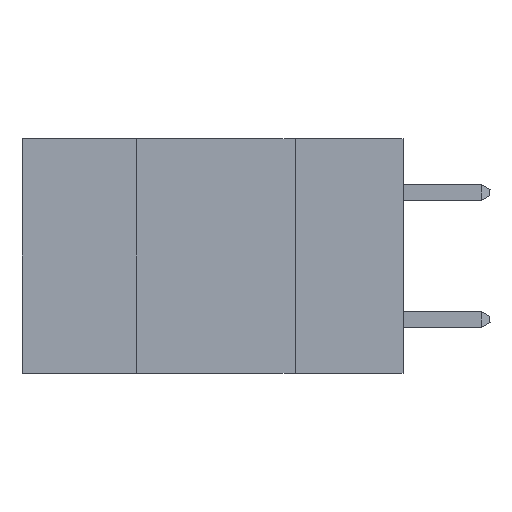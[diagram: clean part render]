
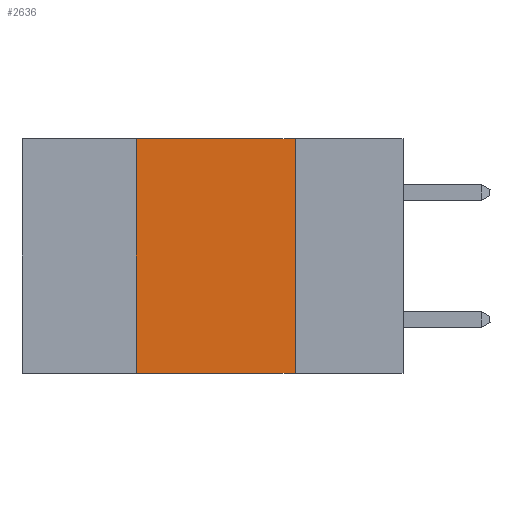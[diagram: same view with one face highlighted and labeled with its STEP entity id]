
A CAD part, left-side view. The second image highlights one B-rep face of the part: STEP entity #2636.
In plain terms, the highlighted planar face has unit normal (-1, 0, 0).
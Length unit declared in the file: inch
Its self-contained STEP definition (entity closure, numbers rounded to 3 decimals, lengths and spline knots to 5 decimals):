
#316 = AXIS2_PLACEMENT_3D ( 'NONE', #5887, #2068, #5934 ) ;
#501 = VERTEX_POINT ( 'NONE', #3597 ) ;
#1115 = CARTESIAN_POINT ( 'NONE',  ( 0., 0.6, -0.37 ) ) ;
#1188 = LINE ( 'NONE', #8768, #4290 ) ;
#1274 = FACE_OUTER_BOUND ( 'NONE', #12156, .T. ) ;
#1864 = VECTOR ( 'NONE', #12861, 39.37008 ) ;
#1935 = ORIENTED_EDGE ( 'NONE', *, *, #4881, .F. ) ;
#2068 = DIRECTION ( 'NONE',  ( 1., 0., 0. ) ) ;
#2636 = ADVANCED_FACE ( 'NONE', ( #1274 ), #11827, .F. ) ;
#2979 = CARTESIAN_POINT ( 'NONE',  ( 0., 0.17, -0.37 ) ) ;
#3360 = VERTEX_POINT ( 'NONE', #2979 ) ;
#3597 = CARTESIAN_POINT ( 'NONE',  ( 0., 0.17, 0. ) ) ;
#3674 = DIRECTION ( 'NONE',  ( 0., -1., 0. ) ) ;
#4053 = VERTEX_POINT ( 'NONE', #8312 ) ;
#4290 = VECTOR ( 'NONE', #3674, 39.37008 ) ;
#4452 = DIRECTION ( 'NONE',  ( 0., 0., -1. ) ) ;
#4752 = CARTESIAN_POINT ( 'NONE',  ( 0., 0.42, 0. ) ) ;
#4881 = EDGE_CURVE ( 'NONE', #12622, #4053, #8793, .T. ) ;
#5273 = VECTOR ( 'NONE', #7553, 39.37008 ) ;
#5887 = CARTESIAN_POINT ( 'NONE',  ( 0., 0.6, 0. ) ) ;
#5934 = DIRECTION ( 'NONE',  ( 0., 0., -1. ) ) ;
#7088 = ORIENTED_EDGE ( 'NONE', *, *, #7168, .F. ) ;
#7168 = EDGE_CURVE ( 'NONE', #4053, #501, #1188, .T. ) ;
#7553 = DIRECTION ( 'NONE',  ( 0., 0., 1. ) ) ;
#7700 = LINE ( 'NONE', #1115, #1864 ) ;
#8312 = CARTESIAN_POINT ( 'NONE',  ( 0., 0.42, 0. ) ) ;
#8448 = ORIENTED_EDGE ( 'NONE', *, *, #9923, .T. ) ;
#8768 = CARTESIAN_POINT ( 'NONE',  ( 0., 0.6, 0. ) ) ;
#8793 = LINE ( 'NONE', #4752, #5273 ) ;
#9602 = EDGE_CURVE ( 'NONE', #501, #3360, #12544, .T. ) ;
#9923 = EDGE_CURVE ( 'NONE', #12622, #3360, #7700, .T. ) ;
#10193 = VECTOR ( 'NONE', #4452, 39.37008 ) ;
#10228 = CARTESIAN_POINT ( 'NONE',  ( 0., 0.17, 0. ) ) ;
#10968 = CARTESIAN_POINT ( 'NONE',  ( 0., 0.42, -0.37 ) ) ;
#11827 = PLANE ( 'NONE',  #316 ) ;
#12156 = EDGE_LOOP ( 'NONE', ( #12296, #7088, #1935, #8448 ) ) ;
#12296 = ORIENTED_EDGE ( 'NONE', *, *, #9602, .F. ) ;
#12544 = LINE ( 'NONE', #10228, #10193 ) ;
#12622 = VERTEX_POINT ( 'NONE', #10968 ) ;
#12861 = DIRECTION ( 'NONE',  ( 0., -1., 0. ) ) ;
